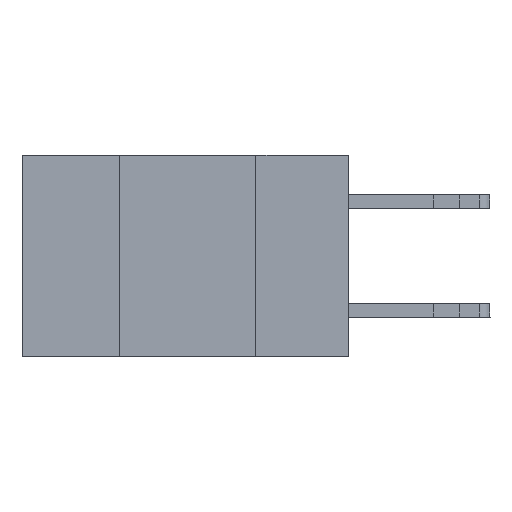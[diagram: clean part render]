
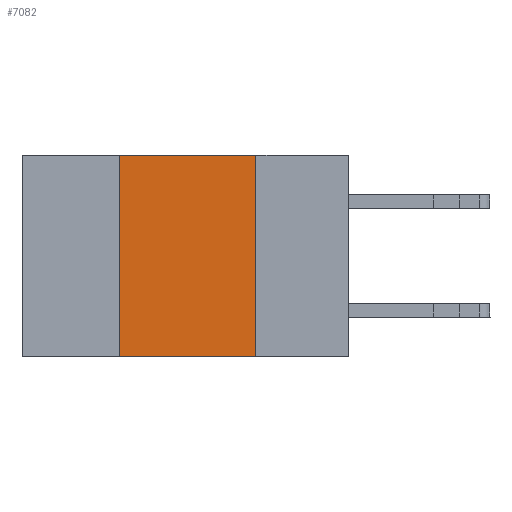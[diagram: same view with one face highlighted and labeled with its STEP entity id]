
A CAD part, left-side view. The second image highlights one B-rep face of the part: STEP entity #7082.
In plain terms, the highlighted planar face has unit normal (-1, 0, 0).
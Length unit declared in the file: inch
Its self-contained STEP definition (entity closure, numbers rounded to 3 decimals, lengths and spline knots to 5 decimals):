
#1834 = DIRECTION ( 'NONE',  ( 0., 0., -1. ) ) ;
#2330 = CARTESIAN_POINT ( 'NONE',  ( 0., 0.6, 0. ) ) ;
#3139 = CARTESIAN_POINT ( 'NONE',  ( 0., 0.42, -0.37 ) ) ;
#4131 = AXIS2_PLACEMENT_3D ( 'NONE', #2330, #15522, #4214 ) ;
#4214 = DIRECTION ( 'NONE',  ( 0., 0., -1. ) ) ;
#4325 = EDGE_CURVE ( 'NONE', #7397, #17346, #9721, .T. ) ;
#5135 = DIRECTION ( 'NONE',  ( 0., -1., 0. ) ) ;
#5713 = LINE ( 'NONE', #16262, #15161 ) ;
#5718 = VECTOR ( 'NONE', #1834, 39.37008 ) ;
#5966 = ORIENTED_EDGE ( 'NONE', *, *, #8950, .F. ) ;
#6346 = ORIENTED_EDGE ( 'NONE', *, *, #7373, .T. ) ;
#6403 = LINE ( 'NONE', #23734, #15215 ) ;
#6452 = EDGE_LOOP ( 'NONE', ( #5966, #15994, #8855, #6346 ) ) ;
#7082 = ADVANCED_FACE ( 'NONE', ( #11692 ), #11790, .F. ) ;
#7373 = EDGE_CURVE ( 'NONE', #7397, #13183, #5713, .T. ) ;
#7397 = VERTEX_POINT ( 'NONE', #3139 ) ;
#8785 = DIRECTION ( 'NONE',  ( 0., -1., 0. ) ) ;
#8855 = ORIENTED_EDGE ( 'NONE', *, *, #4325, .F. ) ;
#8950 = EDGE_CURVE ( 'NONE', #23799, #13183, #11377, .T. ) ;
#9721 = LINE ( 'NONE', #20124, #19126 ) ;
#11377 = LINE ( 'NONE', #18759, #5718 ) ;
#11692 = FACE_OUTER_BOUND ( 'NONE', #6452, .T. ) ;
#11790 = PLANE ( 'NONE',  #4131 ) ;
#13183 = VERTEX_POINT ( 'NONE', #18121 ) ;
#15104 = CARTESIAN_POINT ( 'NONE',  ( 0., 0.42, 0. ) ) ;
#15161 = VECTOR ( 'NONE', #8785, 39.37008 ) ;
#15215 = VECTOR ( 'NONE', #5135, 39.37008 ) ;
#15522 = DIRECTION ( 'NONE',  ( 1., 0., 0. ) ) ;
#15994 = ORIENTED_EDGE ( 'NONE', *, *, #23715, .F. ) ;
#16262 = CARTESIAN_POINT ( 'NONE',  ( 0., 0.6, -0.37 ) ) ;
#16905 = DIRECTION ( 'NONE',  ( 0., 0., 1. ) ) ;
#17346 = VERTEX_POINT ( 'NONE', #15104 ) ;
#18121 = CARTESIAN_POINT ( 'NONE',  ( 0., 0.17, -0.37 ) ) ;
#18759 = CARTESIAN_POINT ( 'NONE',  ( 0., 0.17, 0. ) ) ;
#19126 = VECTOR ( 'NONE', #16905, 39.37008 ) ;
#20124 = CARTESIAN_POINT ( 'NONE',  ( 0., 0.42, 0. ) ) ;
#20416 = CARTESIAN_POINT ( 'NONE',  ( 0., 0.17, 0. ) ) ;
#23715 = EDGE_CURVE ( 'NONE', #17346, #23799, #6403, .T. ) ;
#23734 = CARTESIAN_POINT ( 'NONE',  ( 0., 0.6, 0. ) ) ;
#23799 = VERTEX_POINT ( 'NONE', #20416 ) ;
